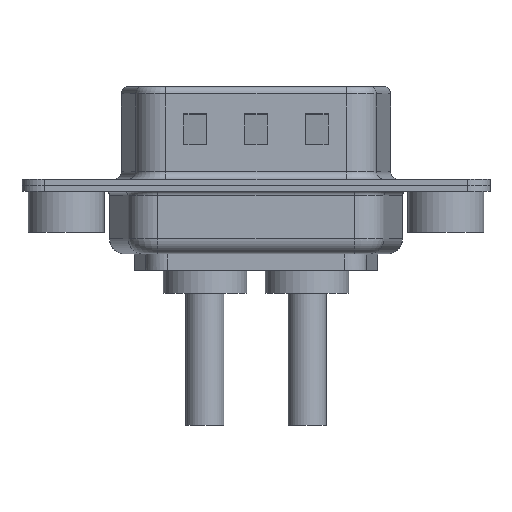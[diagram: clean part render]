
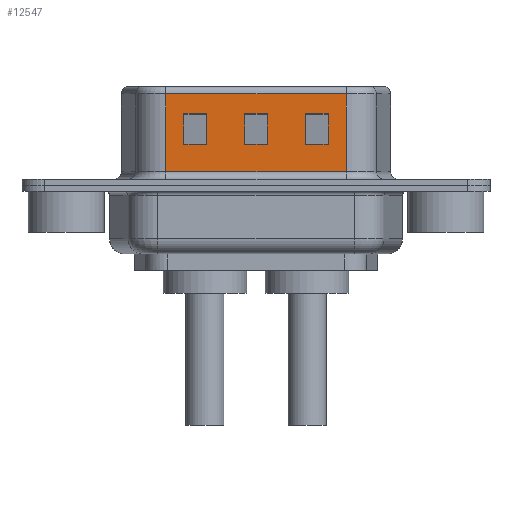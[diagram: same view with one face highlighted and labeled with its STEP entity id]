
A CAD part, front view. The second image highlights one B-rep face of the part: STEP entity #12547.
In plain terms, the highlighted planar face has unit normal (0, -1, 0).
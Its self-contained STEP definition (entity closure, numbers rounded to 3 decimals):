
#19 = VERTEX_POINT ( 'NONE', #14236 ) ;
#96 = VERTEX_POINT ( 'NONE', #2109 ) ;
#119 = FACE_BOUND ( 'NONE', #10164, .T. ) ;
#211 = VERTEX_POINT ( 'NONE', #9053 ) ;
#290 = CARTESIAN_POINT ( 'NONE',  ( 13.25, -4.58, 2.705 ) ) ;
#297 = VECTOR ( 'NONE', #13335, 1000. ) ;
#631 = LINE ( 'NONE', #14411, #9248 ) ;
#960 = PLANE ( 'NONE',  #8973 ) ;
#983 = DIRECTION ( 'NONE',  ( 0., 0., -1. ) ) ;
#1017 = CARTESIAN_POINT ( 'NONE',  ( 13.25, -4.58, 6.52 ) ) ;
#1054 = VERTEX_POINT ( 'NONE', #4967 ) ;
#1095 = EDGE_CURVE ( 'NONE', #1054, #6866, #5342, .T. ) ;
#1128 = EDGE_CURVE ( 'NONE', #7402, #19, #5005, .T. ) ;
#1230 = CARTESIAN_POINT ( 'NONE',  ( 11.75, -4.58, 2.705 ) ) ;
#1424 = VERTEX_POINT ( 'NONE', #13506 ) ;
#1537 = ORIENTED_EDGE ( 'NONE', *, *, #2633, .T. ) ;
#1843 = EDGE_CURVE ( 'NONE', #7716, #7666, #8565, .T. ) ;
#1933 = ORIENTED_EDGE ( 'NONE', *, *, #6352, .T. ) ;
#1934 = ORIENTED_EDGE ( 'NONE', *, *, #14421, .T. ) ;
#2044 = DIRECTION ( 'NONE',  ( 0., 0., -1. ) ) ;
#2109 = CARTESIAN_POINT ( 'NONE',  ( 7.75, -4.58, 4.705 ) ) ;
#2234 = CARTESIAN_POINT ( 'NONE',  ( 17.25, -4.58, 6.52 ) ) ;
#2378 = VECTOR ( 'NONE', #983, 1000. ) ;
#2379 = DIRECTION ( 'NONE',  ( 1., 0., 0. ) ) ;
#2410 = VECTOR ( 'NONE', #8716, 1000. ) ;
#2518 = VERTEX_POINT ( 'NONE', #11581 ) ;
#2633 = EDGE_CURVE ( 'NONE', #6866, #96, #8024, .T. ) ;
#2653 = VECTOR ( 'NONE', #6692, 1000. ) ;
#2822 = ORIENTED_EDGE ( 'NONE', *, *, #10147, .T. ) ;
#2872 = EDGE_LOOP ( 'NONE', ( #7727, #8185, #8909, #2822 ) ) ;
#3238 = DIRECTION ( 'NONE',  ( 0., 1., 0. ) ) ;
#3243 = VECTOR ( 'NONE', #2379, 1000. ) ;
#3325 = LINE ( 'NONE', #5376, #11923 ) ;
#3640 = CARTESIAN_POINT ( 'NONE',  ( 9.25, -4.58, 4.705 ) ) ;
#3753 = LINE ( 'NONE', #9661, #6350 ) ;
#3841 = VECTOR ( 'NONE', #9236, 1000. ) ;
#3865 = VERTEX_POINT ( 'NONE', #1230 ) ;
#4027 = LINE ( 'NONE', #6582, #297 ) ;
#4100 = EDGE_CURVE ( 'NONE', #4667, #7716, #631, .T. ) ;
#4269 = DIRECTION ( 'NONE',  ( -1., 0., 0. ) ) ;
#4561 = LINE ( 'NONE', #4630, #10535 ) ;
#4630 = CARTESIAN_POINT ( 'NONE',  ( 22.45, -4.58, 2.705 ) ) ;
#4667 = VERTEX_POINT ( 'NONE', #5615 ) ;
#4857 = VECTOR ( 'NONE', #5990, 1000. ) ;
#4894 = EDGE_CURVE ( 'NONE', #1424, #2518, #7972, .T. ) ;
#4967 = CARTESIAN_POINT ( 'NONE',  ( 9.25, -4.58, 2.705 ) ) ;
#5005 = LINE ( 'NONE', #6833, #4857 ) ;
#5010 = VECTOR ( 'NONE', #8313, 1000. ) ;
#5053 = VECTOR ( 'NONE', #14072, 1000. ) ;
#5060 = ORIENTED_EDGE ( 'NONE', *, *, #13576, .T. ) ;
#5097 = VERTEX_POINT ( 'NONE', #290 ) ;
#5340 = EDGE_CURVE ( 'NONE', #8047, #1054, #13942, .T. ) ;
#5342 = LINE ( 'NONE', #6901, #2410 ) ;
#5376 = CARTESIAN_POINT ( 'NONE',  ( 18.45, -4.58, 2.705 ) ) ;
#5615 = CARTESIAN_POINT ( 'NONE',  ( 18.45, -4.58, 6.02 ) ) ;
#5651 = DIRECTION ( 'NONE',  ( -1., 0., 0. ) ) ;
#5706 = CARTESIAN_POINT ( 'NONE',  ( 17.25, -4.58, 2.705 ) ) ;
#5719 = ORIENTED_EDGE ( 'NONE', *, *, #1843, .T. ) ;
#5990 = DIRECTION ( 'NONE',  ( 1., 0., 0. ) ) ;
#6003 = LINE ( 'NONE', #2234, #9357 ) ;
#6044 = DIRECTION ( 'NONE',  ( 0., 0., 1. ) ) ;
#6057 = CARTESIAN_POINT ( 'NONE',  ( 6.55, -4.58, 6.02 ) ) ;
#6168 = LINE ( 'NONE', #9051, #3243 ) ;
#6315 = EDGE_CURVE ( 'NONE', #211, #14174, #6003, .T. ) ;
#6350 = VECTOR ( 'NONE', #10778, 1000. ) ;
#6352 = EDGE_CURVE ( 'NONE', #19, #5097, #10935, .T. ) ;
#6405 = CARTESIAN_POINT ( 'NONE',  ( 6.55, -4.58, 0.9 ) ) ;
#6582 = CARTESIAN_POINT ( 'NONE',  ( 18.45, -4.58, 6.52 ) ) ;
#6692 = DIRECTION ( 'NONE',  ( 0., 0., -1. ) ) ;
#6833 = CARTESIAN_POINT ( 'NONE',  ( 18.45, -4.58, 4.705 ) ) ;
#6866 = VERTEX_POINT ( 'NONE', #11307 ) ;
#6901 = CARTESIAN_POINT ( 'NONE',  ( 14.45, -4.58, 2.705 ) ) ;
#6925 = ORIENTED_EDGE ( 'NONE', *, *, #9422, .F. ) ;
#7402 = VERTEX_POINT ( 'NONE', #7963 ) ;
#7577 = ORIENTED_EDGE ( 'NONE', *, *, #9836, .T. ) ;
#7666 = VERTEX_POINT ( 'NONE', #6405 ) ;
#7716 = VERTEX_POINT ( 'NONE', #6057 ) ;
#7727 = ORIENTED_EDGE ( 'NONE', *, *, #6315, .T. ) ;
#7958 = VECTOR ( 'NONE', #8228, 1000. ) ;
#7963 = CARTESIAN_POINT ( 'NONE',  ( 11.75, -4.58, 4.705 ) ) ;
#7972 = LINE ( 'NONE', #8032, #5010 ) ;
#8024 = LINE ( 'NONE', #13727, #5053 ) ;
#8032 = CARTESIAN_POINT ( 'NONE',  ( 15.75, -4.58, 6.52 ) ) ;
#8047 = VERTEX_POINT ( 'NONE', #3640 ) ;
#8090 = CARTESIAN_POINT ( 'NONE',  ( 18.45, -4.58, 0.9 ) ) ;
#8185 = ORIENTED_EDGE ( 'NONE', *, *, #8942, .T. ) ;
#8228 = DIRECTION ( 'NONE',  ( 0., 0., -1. ) ) ;
#8313 = DIRECTION ( 'NONE',  ( 0., 0., 1. ) ) ;
#8366 = ORIENTED_EDGE ( 'NONE', *, *, #4100, .T. ) ;
#8413 = FACE_OUTER_BOUND ( 'NONE', #12674, .T. ) ;
#8565 = LINE ( 'NONE', #13903, #2653 ) ;
#8716 = DIRECTION ( 'NONE',  ( -1., 0., 0. ) ) ;
#8909 = ORIENTED_EDGE ( 'NONE', *, *, #4894, .T. ) ;
#8942 = EDGE_CURVE ( 'NONE', #14174, #1424, #4561, .T. ) ;
#8973 = AXIS2_PLACEMENT_3D ( 'NONE', #11020, #3238, #11060 ) ;
#9051 = CARTESIAN_POINT ( 'NONE',  ( 22.45, -4.58, 4.705 ) ) ;
#9053 = CARTESIAN_POINT ( 'NONE',  ( 17.25, -4.58, 4.705 ) ) ;
#9236 = DIRECTION ( 'NONE',  ( 1., 0., 0. ) ) ;
#9248 = VECTOR ( 'NONE', #5651, 1000. ) ;
#9357 = VECTOR ( 'NONE', #2044, 1000. ) ;
#9378 = ORIENTED_EDGE ( 'NONE', *, *, #5340, .T. ) ;
#9422 = EDGE_CURVE ( 'NONE', #4667, #11929, #4027, .T. ) ;
#9661 = CARTESIAN_POINT ( 'NONE',  ( 14.45, -4.58, 4.705 ) ) ;
#9836 = EDGE_CURVE ( 'NONE', #96, #8047, #3753, .T. ) ;
#10147 = EDGE_CURVE ( 'NONE', #2518, #211, #6168, .T. ) ;
#10164 = EDGE_LOOP ( 'NONE', ( #9378, #13848, #1537, #7577 ) ) ;
#10355 = ORIENTED_EDGE ( 'NONE', *, *, #1128, .T. ) ;
#10535 = VECTOR ( 'NONE', #12457, 1000. ) ;
#10591 = CARTESIAN_POINT ( 'NONE',  ( 11.75, -4.58, 6.52 ) ) ;
#10673 = CARTESIAN_POINT ( 'NONE',  ( 9.25, -4.58, 6.52 ) ) ;
#10675 = LINE ( 'NONE', #10591, #13292 ) ;
#10778 = DIRECTION ( 'NONE',  ( 1., 0., 0. ) ) ;
#10935 = LINE ( 'NONE', #1017, #2378 ) ;
#11020 = CARTESIAN_POINT ( 'NONE',  ( 18.45, -4.58, 6.52 ) ) ;
#11060 = DIRECTION ( 'NONE',  ( 0., 0., 1. ) ) ;
#11307 = CARTESIAN_POINT ( 'NONE',  ( 7.75, -4.58, 2.705 ) ) ;
#11416 = FACE_BOUND ( 'NONE', #2872, .T. ) ;
#11581 = CARTESIAN_POINT ( 'NONE',  ( 15.75, -4.58, 4.705 ) ) ;
#11777 = FACE_BOUND ( 'NONE', #12184, .T. ) ;
#11923 = VECTOR ( 'NONE', #4269, 1000. ) ;
#11929 = VERTEX_POINT ( 'NONE', #12213 ) ;
#12184 = EDGE_LOOP ( 'NONE', ( #10355, #1933, #14176, #1934 ) ) ;
#12213 = CARTESIAN_POINT ( 'NONE',  ( 18.45, -4.58, 0.9 ) ) ;
#12457 = DIRECTION ( 'NONE',  ( -1., 0., 0. ) ) ;
#12547 = ADVANCED_FACE ( 'NONE', ( #119, #11416, #11777, #8413 ), #960, .F. ) ;
#12674 = EDGE_LOOP ( 'NONE', ( #6925, #8366, #5719, #5060 ) ) ;
#12771 = LINE ( 'NONE', #8090, #3841 ) ;
#13292 = VECTOR ( 'NONE', #6044, 1000. ) ;
#13335 = DIRECTION ( 'NONE',  ( 0., 0., -1. ) ) ;
#13506 = CARTESIAN_POINT ( 'NONE',  ( 15.75, -4.58, 2.705 ) ) ;
#13576 = EDGE_CURVE ( 'NONE', #7666, #11929, #12771, .T. ) ;
#13727 = CARTESIAN_POINT ( 'NONE',  ( 7.75, -4.58, 6.52 ) ) ;
#13848 = ORIENTED_EDGE ( 'NONE', *, *, #1095, .T. ) ;
#13903 = CARTESIAN_POINT ( 'NONE',  ( 6.55, -4.58, 6.52 ) ) ;
#13942 = LINE ( 'NONE', #10673, #7958 ) ;
#13954 = EDGE_CURVE ( 'NONE', #5097, #3865, #3325, .T. ) ;
#14072 = DIRECTION ( 'NONE',  ( 0., 0., 1. ) ) ;
#14174 = VERTEX_POINT ( 'NONE', #5706 ) ;
#14176 = ORIENTED_EDGE ( 'NONE', *, *, #13954, .T. ) ;
#14236 = CARTESIAN_POINT ( 'NONE',  ( 13.25, -4.58, 4.705 ) ) ;
#14411 = CARTESIAN_POINT ( 'NONE',  ( 18.45, -4.58, 6.02 ) ) ;
#14421 = EDGE_CURVE ( 'NONE', #3865, #7402, #10675, .T. ) ;
